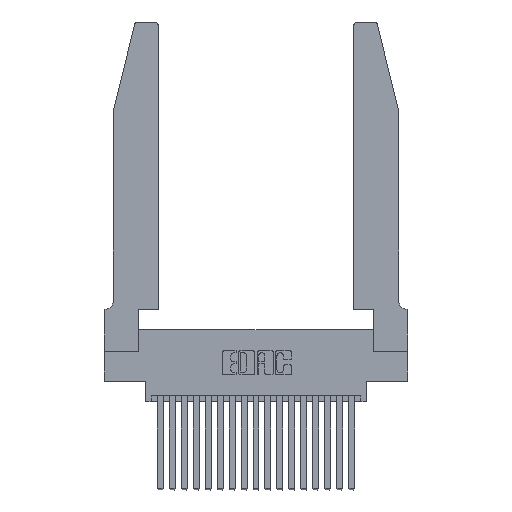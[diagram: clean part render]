
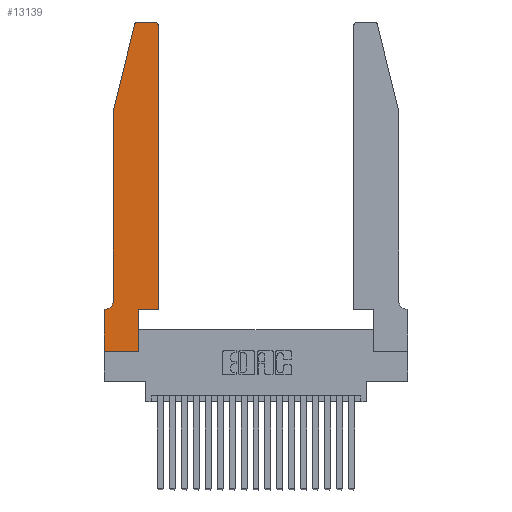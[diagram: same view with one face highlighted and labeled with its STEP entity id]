
A CAD part, top view. The second image highlights one B-rep face of the part: STEP entity #13139.
In plain terms, the highlighted planar face has unit normal (0, 0, 1).
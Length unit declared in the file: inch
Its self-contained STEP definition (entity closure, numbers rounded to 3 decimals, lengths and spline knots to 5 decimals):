
#325 = CARTESIAN_POINT ( 'NONE',  ( 0.2865, 0., 0.37 ) ) ;
#334 = CARTESIAN_POINT ( 'NONE',  ( 0.4205, 2.72, 0.37 ) ) ;
#717 = EDGE_CURVE ( 'NONE', #8313, #15581, #13077, .T. ) ;
#815 = EDGE_CURVE ( 'NONE', #5861, #10083, #15826, .T. ) ;
#1355 = ORIENTED_EDGE ( 'NONE', *, *, #19361, .T. ) ;
#1735 = AXIS2_PLACEMENT_3D ( 'NONE', #12694, #2730, #14288 ) ;
#1785 = ORIENTED_EDGE ( 'NONE', *, *, #3790, .T. ) ;
#2142 = DIRECTION ( 'NONE',  ( 1., 0., 0. ) ) ;
#2165 = CIRCLE ( 'NONE', #14087, 0.07 ) ;
#2309 = VECTOR ( 'NONE', #10363, 39.37008 ) ;
#2407 = ORIENTED_EDGE ( 'NONE', *, *, #14864, .T. ) ;
#2730 = DIRECTION ( 'NONE',  ( 0., 0., 1. ) ) ;
#2833 = FACE_OUTER_BOUND ( 'NONE', #20989, .T. ) ;
#3242 = CARTESIAN_POINT ( 'NONE',  ( 0., 0., 0.37 ) ) ;
#3370 = ORIENTED_EDGE ( 'NONE', *, *, #6360, .T. ) ;
#3578 = VERTEX_POINT ( 'NONE', #3242 ) ;
#3790 = EDGE_CURVE ( 'NONE', #9978, #8313, #6809, .T. ) ;
#3888 = VERTEX_POINT ( 'NONE', #325 ) ;
#4110 = DIRECTION ( 'NONE',  ( 0., 1., 0. ) ) ;
#4269 = CARTESIAN_POINT ( 'NONE',  ( 0.4505, 0.35, 0.37 ) ) ;
#4477 = CARTESIAN_POINT ( 'NONE',  ( 0., 0., 0.37 ) ) ;
#4515 = ORIENTED_EDGE ( 'NONE', *, *, #8229, .T. ) ;
#5523 = ORIENTED_EDGE ( 'NONE', *, *, #815, .T. ) ;
#5541 = DIRECTION ( 'NONE',  ( 1., 0., 0. ) ) ;
#5550 = LINE ( 'NONE', #5863, #18003 ) ;
#5579 = AXIS2_PLACEMENT_3D ( 'NONE', #334, #12167, #2142 ) ;
#5667 = DIRECTION ( 'NONE',  ( 0., 0., -1. ) ) ;
#5861 = VERTEX_POINT ( 'NONE', #15082 ) ;
#5863 = CARTESIAN_POINT ( 'NONE',  ( 0.2865, 0.35, 0.37 ) ) ;
#6118 = CARTESIAN_POINT ( 'NONE',  ( 0.0755, 0.42, 0.37 ) ) ;
#6360 = EDGE_CURVE ( 'NONE', #15581, #13392, #9812, .T. ) ;
#6523 = DIRECTION ( 'NONE',  ( 1., 0., 0. ) ) ;
#6628 = VECTOR ( 'NONE', #6523, 39.37008 ) ;
#6809 = LINE ( 'NONE', #8688, #2309 ) ;
#6943 = DIRECTION ( 'NONE',  ( 0., -1., 0. ) ) ;
#7049 = EDGE_CURVE ( 'NONE', #18667, #17757, #2165, .T. ) ;
#7187 = CARTESIAN_POINT ( 'NONE',  ( 0.0755, 0.35, 0.37 ) ) ;
#7565 = VECTOR ( 'NONE', #5541, 39.37008 ) ;
#7585 = LINE ( 'NONE', #18293, #15243 ) ;
#7717 = VECTOR ( 'NONE', #7751, 39.37008 ) ;
#7751 = DIRECTION ( 'NONE',  ( 0., -1., 0. ) ) ;
#7795 = ORIENTED_EDGE ( 'NONE', *, *, #17429, .T. ) ;
#8229 = EDGE_CURVE ( 'NONE', #17757, #18931, #10840, .T. ) ;
#8242 = LINE ( 'NONE', #4477, #7717 ) ;
#8313 = VERTEX_POINT ( 'NONE', #17069 ) ;
#8534 = VECTOR ( 'NONE', #19608, 39.37008 ) ;
#8688 = CARTESIAN_POINT ( 'NONE',  ( 0.2605, 2.75, 0.37 ) ) ;
#9148 = CARTESIAN_POINT ( 'NONE',  ( 0.25487, 2.72718, 0.37 ) ) ;
#9812 = LINE ( 'NONE', #20085, #14638 ) ;
#9978 = VERTEX_POINT ( 'NONE', #12242 ) ;
#10083 = VERTEX_POINT ( 'NONE', #4269 ) ;
#10363 = DIRECTION ( 'NONE',  ( -1., 0., 0. ) ) ;
#10458 = DIRECTION ( 'NONE',  ( -0.239, -0.971, 0. ) ) ;
#10840 = LINE ( 'NONE', #7187, #18359 ) ;
#11339 = DIRECTION ( 'NONE',  ( 0., 0., 1. ) ) ;
#11966 = LINE ( 'NONE', #12191, #7565 ) ;
#12167 = DIRECTION ( 'NONE',  ( 0., 0., 1. ) ) ;
#12191 = CARTESIAN_POINT ( 'NONE',  ( 0., 0., 0.37 ) ) ;
#12242 = CARTESIAN_POINT ( 'NONE',  ( 0.4205, 2.75, 0.37 ) ) ;
#12694 = CARTESIAN_POINT ( 'NONE',  ( 0., 0.35, 0.37 ) ) ;
#12946 = DIRECTION ( 'NONE',  ( 1., 0., 0. ) ) ;
#12969 = CARTESIAN_POINT ( 'NONE',  ( 0.284, 2.72, 0.37 ) ) ;
#13077 = CIRCLE ( 'NONE', #18821, 0.03 ) ;
#13139 = ADVANCED_FACE ( 'NONE', ( #2833 ), #14212, .T. ) ;
#13392 = VERTEX_POINT ( 'NONE', #19995 ) ;
#13418 = LINE ( 'NONE', #14794, #8534 ) ;
#13888 = VERTEX_POINT ( 'NONE', #21225 ) ;
#14087 = AXIS2_PLACEMENT_3D ( 'NONE', #15444, #5667, #17063 ) ;
#14212 = PLANE ( 'NONE',  #1735 ) ;
#14288 = DIRECTION ( 'NONE',  ( 1., 0., 0. ) ) ;
#14638 = VECTOR ( 'NONE', #10458, 39.37008 ) ;
#14711 = CARTESIAN_POINT ( 'NONE',  ( 0.4505, 0.35, 0.37 ) ) ;
#14794 = CARTESIAN_POINT ( 'NONE',  ( 0.4505, 0.35, 0.37 ) ) ;
#14864 = EDGE_CURVE ( 'NONE', #3888, #5861, #5550, .T. ) ;
#15082 = CARTESIAN_POINT ( 'NONE',  ( 0.2865, 0.35, 0.37 ) ) ;
#15243 = VECTOR ( 'NONE', #6943, 39.37008 ) ;
#15444 = CARTESIAN_POINT ( 'NONE',  ( 0.0055, 0.42, 0.37 ) ) ;
#15581 = VERTEX_POINT ( 'NONE', #9148 ) ;
#15699 = ORIENTED_EDGE ( 'NONE', *, *, #16891, .T. ) ;
#15707 = CIRCLE ( 'NONE', #5579, 0.03 ) ;
#15765 = ORIENTED_EDGE ( 'NONE', *, *, #717, .T. ) ;
#15826 = LINE ( 'NONE', #14711, #6628 ) ;
#15925 = ORIENTED_EDGE ( 'NONE', *, *, #16481, .T. ) ;
#16451 = CARTESIAN_POINT ( 'NONE',  ( 0., 0.35, 0.37 ) ) ;
#16481 = EDGE_CURVE ( 'NONE', #13392, #18667, #7585, .T. ) ;
#16891 = EDGE_CURVE ( 'NONE', #3578, #3888, #11966, .T. ) ;
#17063 = DIRECTION ( 'NONE',  ( -1., 0., 0. ) ) ;
#17069 = CARTESIAN_POINT ( 'NONE',  ( 0.284, 2.75, 0.37 ) ) ;
#17429 = EDGE_CURVE ( 'NONE', #13888, #9978, #15707, .T. ) ;
#17757 = VERTEX_POINT ( 'NONE', #17873 ) ;
#17873 = CARTESIAN_POINT ( 'NONE',  ( 0.0055, 0.35, 0.37 ) ) ;
#18003 = VECTOR ( 'NONE', #4110, 39.37008 ) ;
#18081 = ORIENTED_EDGE ( 'NONE', *, *, #7049, .T. ) ;
#18192 = EDGE_CURVE ( 'NONE', #10083, #13888, #13418, .T. ) ;
#18287 = ORIENTED_EDGE ( 'NONE', *, *, #18192, .T. ) ;
#18293 = CARTESIAN_POINT ( 'NONE',  ( 0.0755, 2., 0.37 ) ) ;
#18359 = VECTOR ( 'NONE', #18528, 39.37008 ) ;
#18528 = DIRECTION ( 'NONE',  ( -1., 0., 0. ) ) ;
#18667 = VERTEX_POINT ( 'NONE', #6118 ) ;
#18821 = AXIS2_PLACEMENT_3D ( 'NONE', #12969, #11339, #12946 ) ;
#18931 = VERTEX_POINT ( 'NONE', #16451 ) ;
#19361 = EDGE_CURVE ( 'NONE', #18931, #3578, #8242, .T. ) ;
#19608 = DIRECTION ( 'NONE',  ( 0., 1., 0. ) ) ;
#19995 = CARTESIAN_POINT ( 'NONE',  ( 0.0755, 2., 0.37 ) ) ;
#20085 = CARTESIAN_POINT ( 'NONE',  ( 0.0755, 2., 0.37 ) ) ;
#20989 = EDGE_LOOP ( 'NONE', ( #1785, #15765, #3370, #15925, #18081, #4515, #1355, #15699, #2407, #5523, #18287, #7795 ) ) ;
#21225 = CARTESIAN_POINT ( 'NONE',  ( 0.4505, 2.72, 0.37 ) ) ;
